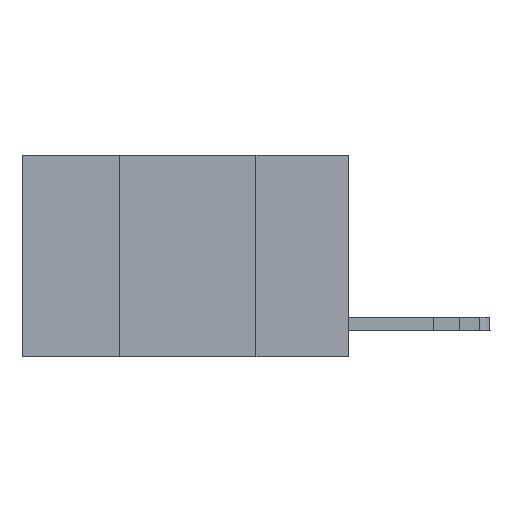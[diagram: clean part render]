
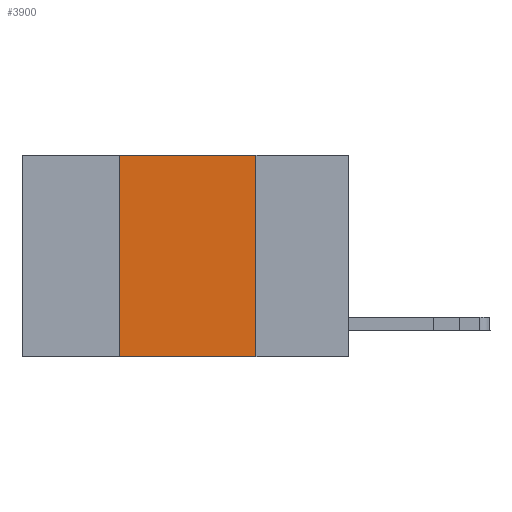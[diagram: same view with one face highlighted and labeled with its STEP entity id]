
A CAD part, left-side view. The second image highlights one B-rep face of the part: STEP entity #3900.
In plain terms, the highlighted planar face has unit normal (-1, 0, 0).
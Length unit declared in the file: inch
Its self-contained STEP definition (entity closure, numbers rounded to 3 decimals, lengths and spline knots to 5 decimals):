
#56 = AXIS2_PLACEMENT_3D ( 'NONE', #13911, #10007, #15094 ) ;
#298 = VERTEX_POINT ( 'NONE', #15968 ) ;
#519 = EDGE_CURVE ( 'NONE', #298, #11697, #7491, .T. ) ;
#1955 = VECTOR ( 'NONE', #14521, 39.37008 ) ;
#1967 = DIRECTION ( 'NONE',  ( 0., -1., 0. ) ) ;
#2627 = FACE_OUTER_BOUND ( 'NONE', #11113, .T. ) ;
#3062 = VECTOR ( 'NONE', #7201, 39.37008 ) ;
#3900 = ADVANCED_FACE ( 'NONE', ( #2627 ), #11253, .F. ) ;
#4942 = CARTESIAN_POINT ( 'NONE',  ( 0., 0.17, 0. ) ) ;
#5731 = EDGE_CURVE ( 'NONE', #5765, #11697, #14743, .T. ) ;
#5765 = VERTEX_POINT ( 'NONE', #15083 ) ;
#6028 = ORIENTED_EDGE ( 'NONE', *, *, #15515, .F. ) ;
#6057 = CARTESIAN_POINT ( 'NONE',  ( 0., 0.42, 0. ) ) ;
#6958 = LINE ( 'NONE', #13340, #8983 ) ;
#7201 = DIRECTION ( 'NONE',  ( 0., 0., -1. ) ) ;
#7491 = LINE ( 'NONE', #14025, #12248 ) ;
#7646 = ORIENTED_EDGE ( 'NONE', *, *, #519, .T. ) ;
#8700 = CARTESIAN_POINT ( 'NONE',  ( 0., 0.17, -0.37 ) ) ;
#8983 = VECTOR ( 'NONE', #1967, 39.37008 ) ;
#9443 = CARTESIAN_POINT ( 'NONE',  ( 0., 0.42, 0. ) ) ;
#10007 = DIRECTION ( 'NONE',  ( 1., 0., 0. ) ) ;
#11002 = LINE ( 'NONE', #9443, #1955 ) ;
#11113 = EDGE_LOOP ( 'NONE', ( #11294, #6028, #13073, #7646 ) ) ;
#11253 = PLANE ( 'NONE',  #56 ) ;
#11286 = DIRECTION ( 'NONE',  ( 0., -1., 0. ) ) ;
#11294 = ORIENTED_EDGE ( 'NONE', *, *, #5731, .F. ) ;
#11589 = VERTEX_POINT ( 'NONE', #6057 ) ;
#11697 = VERTEX_POINT ( 'NONE', #8700 ) ;
#12248 = VECTOR ( 'NONE', #11286, 39.37008 ) ;
#13073 = ORIENTED_EDGE ( 'NONE', *, *, #14200, .F. ) ;
#13340 = CARTESIAN_POINT ( 'NONE',  ( 0., 0.6, 0. ) ) ;
#13911 = CARTESIAN_POINT ( 'NONE',  ( 0., 0.6, 0. ) ) ;
#14025 = CARTESIAN_POINT ( 'NONE',  ( 0., 0.6, -0.37 ) ) ;
#14200 = EDGE_CURVE ( 'NONE', #298, #11589, #11002, .T. ) ;
#14521 = DIRECTION ( 'NONE',  ( 0., 0., 1. ) ) ;
#14743 = LINE ( 'NONE', #4942, #3062 ) ;
#15083 = CARTESIAN_POINT ( 'NONE',  ( 0., 0.17, 0. ) ) ;
#15094 = DIRECTION ( 'NONE',  ( 0., 0., -1. ) ) ;
#15515 = EDGE_CURVE ( 'NONE', #11589, #5765, #6958, .T. ) ;
#15968 = CARTESIAN_POINT ( 'NONE',  ( 0., 0.42, -0.37 ) ) ;
